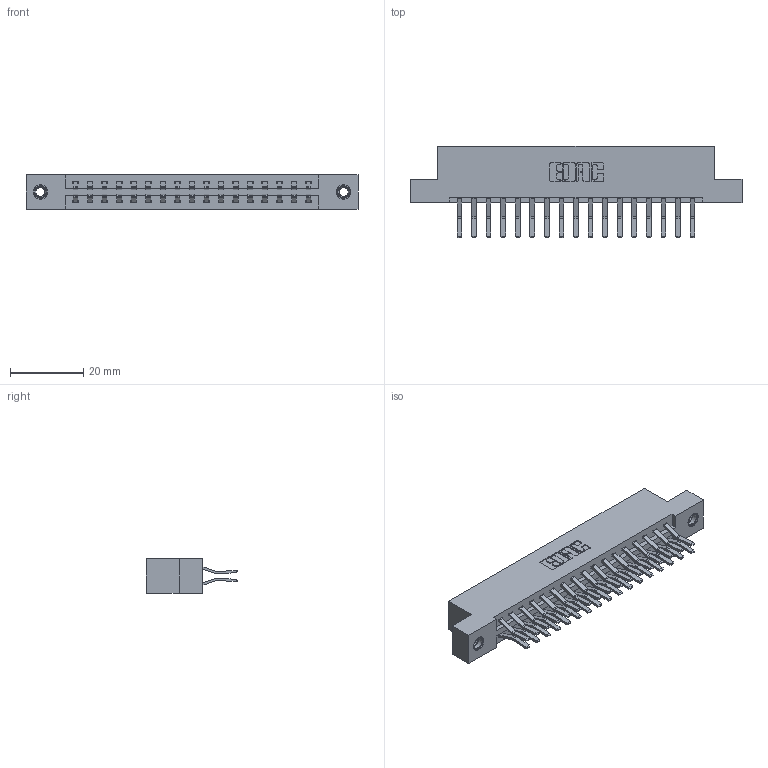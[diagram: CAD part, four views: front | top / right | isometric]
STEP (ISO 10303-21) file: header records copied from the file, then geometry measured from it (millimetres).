
FILE_DESCRIPTION (( 'STEP AP203' ), '1' );
FILE_NAME ('337-034-560-207.STEP', '2018-08-07T19:36:57', ( '' ), ( '' ), 'SwSTEP 2.0', 'SolidWorks 2016', '' );
FILE_SCHEMA (( 'CONFIG_CONTROL_DESIGN' ));
Length unit declared in the file: inch
Products named in the file (4): 337 Part_Flush Mounting Lugs - 0.156 Dia-TI; 345-292-001_560 Tail; 345-250-001_345-250-005-103; 337-034-560-207
Assembly tree (37 placements, depth 2):
  337-034-560-207
    337 Part_Flush Mounting Lugs - 0.156 Dia-TI
    345-292-001_560 Tail  x34
    345-250-001_345-250-005-103  x2
Bounding box: 90.37 x 24.78 x 9.4 mm (x, y, z)
Volume: 9400.8 mm3; surface area: 11065.7 mm2
Topology: 37 solids, 37 shells, 2078 faces, 6125 edges, 4030 vertices
Faces by surface type: plane 1394, cylinder 668, cone 12, torus 4
Entity records: 17688 total; most frequent: CARTESIAN_POINT 2981, ORIENTED_EDGE 2910, DIRECTION 2617, EDGE_CURVE 1455, VECTOR 1303, LINE 1303, VERTEX_POINT 964, AXIS2_PLACEMENT_3D 657
